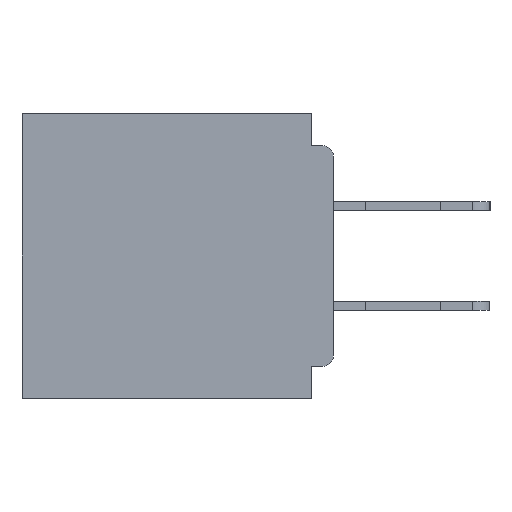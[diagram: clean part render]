
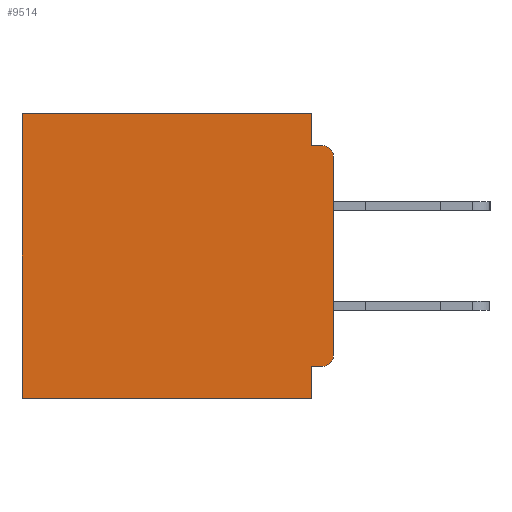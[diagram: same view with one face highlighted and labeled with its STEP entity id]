
A CAD part, left-side view. The second image highlights one B-rep face of the part: STEP entity #9514.
In plain terms, the highlighted planar face has unit normal (-1, 0, 0).
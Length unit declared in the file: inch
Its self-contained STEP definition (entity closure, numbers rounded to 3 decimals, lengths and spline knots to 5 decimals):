
#143 = VERTEX_POINT ( 'NONE', #17223 ) ;
#549 = EDGE_CURVE ( 'NONE', #54350, #36320, #49053, .T. ) ;
#1308 = AXIS2_PLACEMENT_3D ( 'NONE', #38068, #10712, #42697 ) ;
#2645 = DIRECTION ( 'NONE',  ( 0., 0., -1. ) ) ;
#2735 = FACE_OUTER_BOUND ( 'NONE', #33483, .T. ) ;
#3983 = CARTESIAN_POINT ( 'NONE',  ( 0.3, 0., 0. ) ) ;
#4093 = CARTESIAN_POINT ( 'NONE',  ( 0.3, 0.031, 0. ) ) ;
#7264 = ORIENTED_EDGE ( 'NONE', *, *, #39873, .T. ) ;
#7615 = CIRCLE ( 'NONE', #50053, 0.015 ) ;
#7973 = ORIENTED_EDGE ( 'NONE', *, *, #55267, .F. ) ;
#8108 = EDGE_CURVE ( 'NONE', #42884, #36320, #13451, .T. ) ;
#8803 = CARTESIAN_POINT ( 'NONE',  ( 0.3, 0., -0.34 ) ) ;
#9514 = ADVANCED_FACE ( 'NONE', ( #2735 ), #16563, .F. ) ;
#9647 = EDGE_CURVE ( 'NONE', #50567, #18033, #44187, .T. ) ;
#10361 = LINE ( 'NONE', #30013, #59023 ) ;
#10712 = DIRECTION ( 'NONE',  ( -1., 0., 0. ) ) ;
#11568 = ORIENTED_EDGE ( 'NONE', *, *, #24180, .F. ) ;
#12386 = VECTOR ( 'NONE', #19322, 39.37008 ) ;
#13224 = LINE ( 'NONE', #45134, #23954 ) ;
#13451 = CIRCLE ( 'NONE', #1308, 0.015 ) ;
#14938 = LINE ( 'NONE', #17080, #25685 ) ;
#16563 = PLANE ( 'NONE',  #44303 ) ;
#16670 = CARTESIAN_POINT ( 'NONE',  ( 0.3, 0.031, 0. ) ) ;
#17080 = CARTESIAN_POINT ( 'NONE',  ( 0.3, 0.437, -0.4 ) ) ;
#17096 = CARTESIAN_POINT ( 'NONE',  ( 0.3, 0., -0.355 ) ) ;
#17182 = CARTESIAN_POINT ( 'NONE',  ( 0.3, 0.031, -0.045 ) ) ;
#17223 = CARTESIAN_POINT ( 'NONE',  ( 0.3, 0.437, -0.4 ) ) ;
#17595 = CARTESIAN_POINT ( 'NONE',  ( 0.3, 0.015, -0.34 ) ) ;
#18033 = VERTEX_POINT ( 'NONE', #56125 ) ;
#18825 = EDGE_CURVE ( 'NONE', #35004, #57185, #10361, .T. ) ;
#18848 = LINE ( 'NONE', #16670, #43173 ) ;
#19322 = DIRECTION ( 'NONE',  ( 0., 1., 0. ) ) ;
#19864 = VECTOR ( 'NONE', #22374, 39.37008 ) ;
#20722 = ORIENTED_EDGE ( 'NONE', *, *, #549, .F. ) ;
#21375 = DIRECTION ( 'NONE',  ( 0., 0., -1. ) ) ;
#22230 = DIRECTION ( 'NONE',  ( 0., 0., -1. ) ) ;
#22374 = DIRECTION ( 'NONE',  ( 0., 1., 0. ) ) ;
#23934 = VECTOR ( 'NONE', #49067, 39.37008 ) ;
#23954 = VECTOR ( 'NONE', #26907, 39.37008 ) ;
#24115 = CARTESIAN_POINT ( 'NONE',  ( 0.3, 0., -0.4 ) ) ;
#24180 = EDGE_CURVE ( 'NONE', #42884, #39919, #13224, .T. ) ;
#24980 = EDGE_CURVE ( 'NONE', #50567, #54350, #18848, .T. ) ;
#25685 = VECTOR ( 'NONE', #44693, 39.37008 ) ;
#26907 = DIRECTION ( 'NONE',  ( 0., 0., -1. ) ) ;
#28642 = CARTESIAN_POINT ( 'NONE',  ( 0.3, 0.015, -0.355 ) ) ;
#30013 = CARTESIAN_POINT ( 'NONE',  ( 0.3, 0.031, -0.4 ) ) ;
#33483 = EDGE_LOOP ( 'NONE', ( #11568, #36766, #20722, #59183, #55678, #47107, #7973, #57304, #42944, #7264 ) ) ;
#34950 = CARTESIAN_POINT ( 'NONE',  ( 0.3, 0., -0.4 ) ) ;
#35004 = VERTEX_POINT ( 'NONE', #47612 ) ;
#36320 = VERTEX_POINT ( 'NONE', #37407 ) ;
#36766 = ORIENTED_EDGE ( 'NONE', *, *, #8108, .T. ) ;
#37407 = CARTESIAN_POINT ( 'NONE',  ( 0.3, 0.015, -0.045 ) ) ;
#37912 = CARTESIAN_POINT ( 'NONE',  ( 0.3, 0.031, -0.4 ) ) ;
#38068 = CARTESIAN_POINT ( 'NONE',  ( 0.3, 0.015, -0.06 ) ) ;
#39436 = DIRECTION ( 'NONE',  ( 0., 0., -1. ) ) ;
#39873 = EDGE_CURVE ( 'NONE', #41484, #39919, #7615, .T. ) ;
#39919 = VERTEX_POINT ( 'NONE', #8803 ) ;
#41484 = VERTEX_POINT ( 'NONE', #28642 ) ;
#41833 = EDGE_CURVE ( 'NONE', #41484, #35004, #58973, .T. ) ;
#42697 = DIRECTION ( 'NONE',  ( 0., 0., -1. ) ) ;
#42884 = VERTEX_POINT ( 'NONE', #57397 ) ;
#42944 = ORIENTED_EDGE ( 'NONE', *, *, #41833, .F. ) ;
#43173 = VECTOR ( 'NONE', #39436, 39.37008 ) ;
#44187 = LINE ( 'NONE', #3983, #19864 ) ;
#44303 = AXIS2_PLACEMENT_3D ( 'NONE', #34950, #48739, #21375 ) ;
#44693 = DIRECTION ( 'NONE',  ( 0., 0., -1. ) ) ;
#45134 = CARTESIAN_POINT ( 'NONE',  ( 0.3, 0., -0.4 ) ) ;
#47107 = ORIENTED_EDGE ( 'NONE', *, *, #50506, .T. ) ;
#47612 = CARTESIAN_POINT ( 'NONE',  ( 0.3, 0.031, -0.355 ) ) ;
#47626 = VECTOR ( 'NONE', #48892, 39.37008 ) ;
#48739 = DIRECTION ( 'NONE',  ( 1., 0., 0. ) ) ;
#48858 = LINE ( 'NONE', #24115, #12386 ) ;
#48892 = DIRECTION ( 'NONE',  ( 0., -1., 0. ) ) ;
#49053 = LINE ( 'NONE', #49219, #47626 ) ;
#49067 = DIRECTION ( 'NONE',  ( 0., 1., 0. ) ) ;
#49219 = CARTESIAN_POINT ( 'NONE',  ( 0.3, 0., -0.045 ) ) ;
#49575 = DIRECTION ( 'NONE',  ( -1., 0., 0. ) ) ;
#50053 = AXIS2_PLACEMENT_3D ( 'NONE', #17595, #49575, #22230 ) ;
#50506 = EDGE_CURVE ( 'NONE', #18033, #143, #14938, .T. ) ;
#50567 = VERTEX_POINT ( 'NONE', #4093 ) ;
#54350 = VERTEX_POINT ( 'NONE', #17182 ) ;
#55267 = EDGE_CURVE ( 'NONE', #57185, #143, #48858, .T. ) ;
#55678 = ORIENTED_EDGE ( 'NONE', *, *, #9647, .T. ) ;
#56125 = CARTESIAN_POINT ( 'NONE',  ( 0.3, 0.437, 0. ) ) ;
#57185 = VERTEX_POINT ( 'NONE', #37912 ) ;
#57304 = ORIENTED_EDGE ( 'NONE', *, *, #18825, .F. ) ;
#57397 = CARTESIAN_POINT ( 'NONE',  ( 0.3, 0., -0.06 ) ) ;
#58973 = LINE ( 'NONE', #17096, #23934 ) ;
#59023 = VECTOR ( 'NONE', #2645, 39.37008 ) ;
#59183 = ORIENTED_EDGE ( 'NONE', *, *, #24980, .F. ) ;
